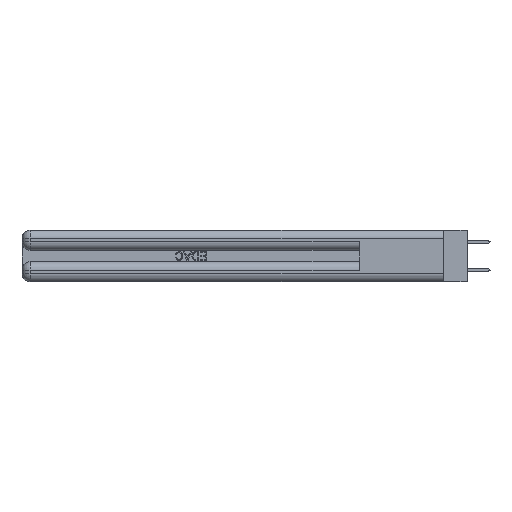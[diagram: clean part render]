
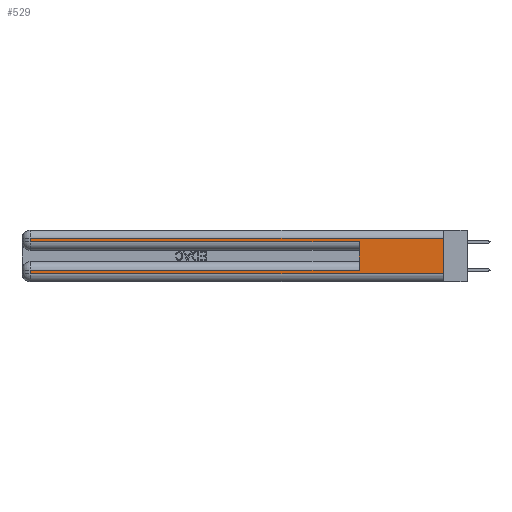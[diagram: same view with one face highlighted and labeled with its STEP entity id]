
A CAD part, left-side view. The second image highlights one B-rep face of the part: STEP entity #529.
In plain terms, the highlighted planar face has unit normal (-1, 0, 0).
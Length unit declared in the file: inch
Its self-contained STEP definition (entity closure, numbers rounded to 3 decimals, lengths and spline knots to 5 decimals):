
#57 = CARTESIAN_POINT ( 'NONE',  ( 0., 2.94, 0.37 ) ) ;
#190 = DIRECTION ( 'NONE',  ( 0., 1., 0. ) ) ;
#529 = ADVANCED_FACE ( 'NONE', ( #42235 ), #29334, .F. ) ;
#942 = DIRECTION ( 'NONE',  ( 0., 1., 0. ) ) ;
#1326 = EDGE_CURVE ( 'NONE', #6780, #11451, #15358, .T. ) ;
#1613 = DIRECTION ( 'NONE',  ( 0., -1., 0. ) ) ;
#1802 = VECTOR ( 'NONE', #11422, 39.37008 ) ;
#3755 = LINE ( 'NONE', #8259, #20174 ) ;
#3759 = LINE ( 'NONE', #22557, #24512 ) ;
#3882 = DIRECTION ( 'NONE',  ( 0., -1., 0. ) ) ;
#4654 = VERTEX_POINT ( 'NONE', #34111 ) ;
#5505 = EDGE_CURVE ( 'NONE', #32529, #4654, #29665, .T. ) ;
#5781 = ORIENTED_EDGE ( 'NONE', *, *, #19633, .F. ) ;
#6314 = VERTEX_POINT ( 'NONE', #8602 ) ;
#6665 = LINE ( 'NONE', #35183, #7755 ) ;
#6780 = VERTEX_POINT ( 'NONE', #7491 ) ;
#7491 = CARTESIAN_POINT ( 'NONE',  ( 0., 2.94, 0.085 ) ) ;
#7755 = VECTOR ( 'NONE', #3882, 39.37008 ) ;
#7801 = CARTESIAN_POINT ( 'NONE',  ( 0., 0.6, 0.285 ) ) ;
#8259 = CARTESIAN_POINT ( 'NONE',  ( 0., 0., 0.37 ) ) ;
#8602 = CARTESIAN_POINT ( 'NONE',  ( 0., 0., 0.31 ) ) ;
#8932 = CARTESIAN_POINT ( 'NONE',  ( 0., 2.94, 0.06 ) ) ;
#9446 = ORIENTED_EDGE ( 'NONE', *, *, #37815, .T. ) ;
#11422 = DIRECTION ( 'NONE',  ( 0., 0., -1. ) ) ;
#11451 = VERTEX_POINT ( 'NONE', #8932 ) ;
#11793 = DIRECTION ( 'NONE',  ( 0., 0., -1. ) ) ;
#11966 = DIRECTION ( 'NONE',  ( 0., 0., -1. ) ) ;
#12709 = LINE ( 'NONE', #25345, #13813 ) ;
#12833 = LINE ( 'NONE', #24601, #30276 ) ;
#13263 = CARTESIAN_POINT ( 'NONE',  ( 0., 0.6, 0.145 ) ) ;
#13409 = ORIENTED_EDGE ( 'NONE', *, *, #28742, .T. ) ;
#13813 = VECTOR ( 'NONE', #942, 39.37008 ) ;
#14053 = VERTEX_POINT ( 'NONE', #7801 ) ;
#14262 = VECTOR ( 'NONE', #24461, 39.37008 ) ;
#15358 = LINE ( 'NONE', #57, #14262 ) ;
#15560 = ORIENTED_EDGE ( 'NONE', *, *, #32196, .F. ) ;
#16565 = EDGE_CURVE ( 'NONE', #6314, #32529, #12709, .T. ) ;
#18498 = VECTOR ( 'NONE', #20295, 39.37008 ) ;
#18899 = CARTESIAN_POINT ( 'NONE',  ( 0., 0.6, 0.085 ) ) ;
#19633 = EDGE_CURVE ( 'NONE', #37340, #14053, #27746, .T. ) ;
#20174 = VECTOR ( 'NONE', #11793, 39.37008 ) ;
#20295 = DIRECTION ( 'NONE',  ( 0., 0., 1. ) ) ;
#22309 = CARTESIAN_POINT ( 'NONE',  ( 0., 0., 0.06 ) ) ;
#22557 = CARTESIAN_POINT ( 'NONE',  ( 0., 0., 0.285 ) ) ;
#24404 = CARTESIAN_POINT ( 'NONE',  ( 0., 2.94, 0.31 ) ) ;
#24461 = DIRECTION ( 'NONE',  ( 0., 0., -1. ) ) ;
#24512 = VECTOR ( 'NONE', #1613, 39.37008 ) ;
#24601 = CARTESIAN_POINT ( 'NONE',  ( 0., 0., 0.085 ) ) ;
#25130 = ORIENTED_EDGE ( 'NONE', *, *, #5505, .T. ) ;
#25265 = CARTESIAN_POINT ( 'NONE',  ( 0., 2.94, 0.37 ) ) ;
#25345 = CARTESIAN_POINT ( 'NONE',  ( 0., 0., 0.31 ) ) ;
#27626 = EDGE_LOOP ( 'NONE', ( #15560, #27860, #25130, #39602, #5781, #13409, #42870, #9446 ) ) ;
#27746 = LINE ( 'NONE', #13263, #18498 ) ;
#27860 = ORIENTED_EDGE ( 'NONE', *, *, #16565, .T. ) ;
#28742 = EDGE_CURVE ( 'NONE', #37340, #6780, #12833, .T. ) ;
#29184 = AXIS2_PLACEMENT_3D ( 'NONE', #42925, #32759, #11966 ) ;
#29334 = PLANE ( 'NONE',  #29184 ) ;
#29665 = LINE ( 'NONE', #25265, #1802 ) ;
#30276 = VECTOR ( 'NONE', #190, 39.37008 ) ;
#32196 = EDGE_CURVE ( 'NONE', #6314, #36546, #3755, .T. ) ;
#32529 = VERTEX_POINT ( 'NONE', #24404 ) ;
#32759 = DIRECTION ( 'NONE',  ( 1., 0., 0. ) ) ;
#32862 = EDGE_CURVE ( 'NONE', #4654, #14053, #3759, .T. ) ;
#34111 = CARTESIAN_POINT ( 'NONE',  ( 0., 2.94, 0.285 ) ) ;
#35183 = CARTESIAN_POINT ( 'NONE',  ( 0., 0., 0.06 ) ) ;
#36546 = VERTEX_POINT ( 'NONE', #22309 ) ;
#37340 = VERTEX_POINT ( 'NONE', #18899 ) ;
#37815 = EDGE_CURVE ( 'NONE', #11451, #36546, #6665, .T. ) ;
#39602 = ORIENTED_EDGE ( 'NONE', *, *, #32862, .T. ) ;
#42235 = FACE_OUTER_BOUND ( 'NONE', #27626, .T. ) ;
#42870 = ORIENTED_EDGE ( 'NONE', *, *, #1326, .T. ) ;
#42925 = CARTESIAN_POINT ( 'NONE',  ( 0., 0., 0.37 ) ) ;
